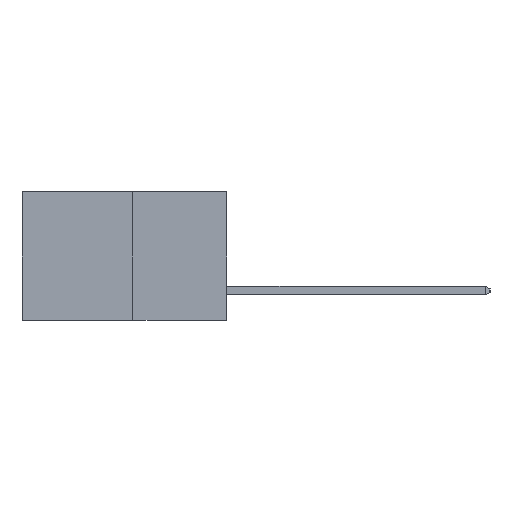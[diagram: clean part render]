
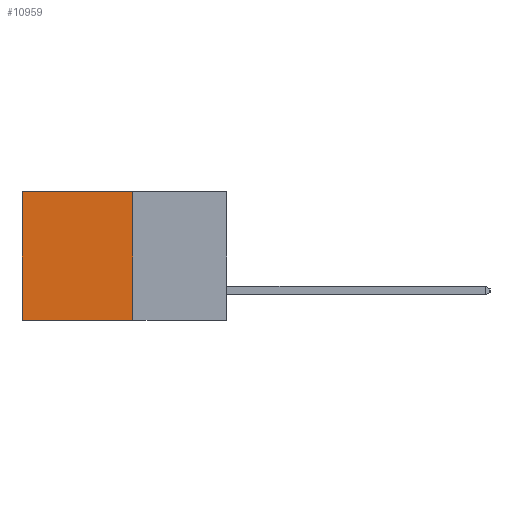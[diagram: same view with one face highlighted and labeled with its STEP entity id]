
A CAD part, left-side view. The second image highlights one B-rep face of the part: STEP entity #10959.
In plain terms, the highlighted planar face has unit normal (-1, 0, 0).
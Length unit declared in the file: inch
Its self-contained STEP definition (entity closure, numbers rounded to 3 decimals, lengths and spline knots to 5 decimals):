
#69 = CARTESIAN_POINT ( 'NONE',  ( 0.277, 0.27, 0. ) ) ;
#223 = LINE ( 'NONE', #18508, #4888 ) ;
#405 = VERTEX_POINT ( 'NONE', #14200 ) ;
#490 = ORIENTED_EDGE ( 'NONE', *, *, #25403, .F. ) ;
#1418 = ORIENTED_EDGE ( 'NONE', *, *, #15824, .T. ) ;
#1825 = CARTESIAN_POINT ( 'NONE',  ( 0.277, 0.27, -0.37 ) ) ;
#2123 = PLANE ( 'NONE',  #24946 ) ;
#3043 = CARTESIAN_POINT ( 'NONE',  ( 0.277, 0.27, -0.37 ) ) ;
#3156 = DIRECTION ( 'NONE',  ( 0., 0., -1. ) ) ;
#3737 = EDGE_CURVE ( 'NONE', #15310, #24577, #22541, .T. ) ;
#4137 = CARTESIAN_POINT ( 'NONE',  ( 0.277, 0.27, -0.37 ) ) ;
#4888 = VECTOR ( 'NONE', #8663, 39.37008 ) ;
#6165 = DIRECTION ( 'NONE',  ( 0., 0., -1. ) ) ;
#8257 = FACE_OUTER_BOUND ( 'NONE', #23707, .T. ) ;
#8663 = DIRECTION ( 'NONE',  ( 0., 1., 0. ) ) ;
#9712 = VECTOR ( 'NONE', #13922, 39.37008 ) ;
#10959 = ADVANCED_FACE ( 'NONE', ( #8257 ), #2123, .F. ) ;
#12098 = ORIENTED_EDGE ( 'NONE', *, *, #3737, .F. ) ;
#12189 = VECTOR ( 'NONE', #13984, 39.37008 ) ;
#13131 = EDGE_CURVE ( 'NONE', #405, #24577, #18968, .T. ) ;
#13164 = CARTESIAN_POINT ( 'NONE',  ( 0.277, 0.59, -0.37 ) ) ;
#13618 = ORIENTED_EDGE ( 'NONE', *, *, #13131, .T. ) ;
#13922 = DIRECTION ( 'NONE',  ( 0., 0., -1. ) ) ;
#13984 = DIRECTION ( 'NONE',  ( 0., 1., 0. ) ) ;
#14200 = CARTESIAN_POINT ( 'NONE',  ( 0.277, 0.59, 0. ) ) ;
#14992 = LINE ( 'NONE', #1825, #9712 ) ;
#15310 = VERTEX_POINT ( 'NONE', #3043 ) ;
#15824 = EDGE_CURVE ( 'NONE', #20563, #405, #223, .T. ) ;
#17342 = CARTESIAN_POINT ( 'NONE',  ( 0.277, 0.27, -0.37 ) ) ;
#18073 = DIRECTION ( 'NONE',  ( 1., 0., 0. ) ) ;
#18508 = CARTESIAN_POINT ( 'NONE',  ( 0.277, 0.27, 0. ) ) ;
#18968 = LINE ( 'NONE', #13164, #23510 ) ;
#20563 = VERTEX_POINT ( 'NONE', #69 ) ;
#22541 = LINE ( 'NONE', #17342, #12189 ) ;
#23510 = VECTOR ( 'NONE', #3156, 39.37008 ) ;
#23707 = EDGE_LOOP ( 'NONE', ( #13618, #12098, #490, #1418 ) ) ;
#24577 = VERTEX_POINT ( 'NONE', #24784 ) ;
#24784 = CARTESIAN_POINT ( 'NONE',  ( 0.277, 0.59, -0.37 ) ) ;
#24946 = AXIS2_PLACEMENT_3D ( 'NONE', #4137, #18073, #6165 ) ;
#25403 = EDGE_CURVE ( 'NONE', #20563, #15310, #14992, .T. ) ;
